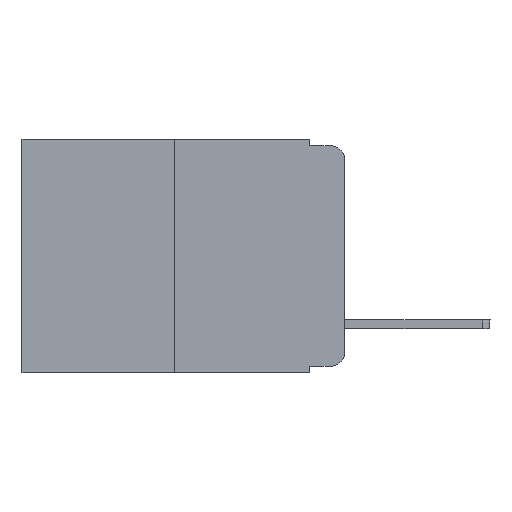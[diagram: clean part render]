
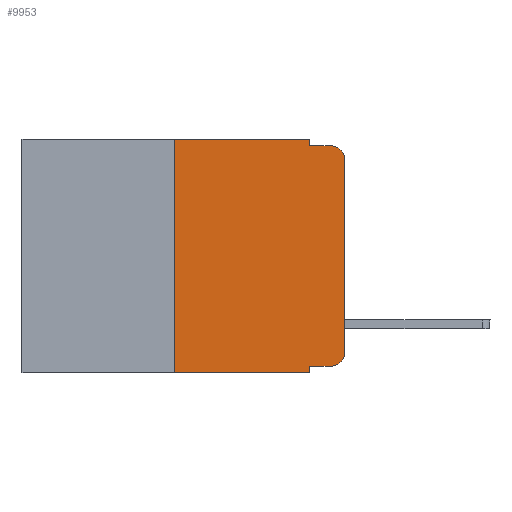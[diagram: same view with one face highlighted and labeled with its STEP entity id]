
A CAD part, left-side view. The second image highlights one B-rep face of the part: STEP entity #9953.
In plain terms, the highlighted planar face has unit normal (-1, 0, 0).
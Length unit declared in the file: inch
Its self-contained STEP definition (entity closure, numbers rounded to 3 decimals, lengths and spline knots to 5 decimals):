
#161 = CARTESIAN_POINT ( 'NONE',  ( 0., 0.473, 0. ) ) ;
#421 = DIRECTION ( 'NONE',  ( 0., -1., 0. ) ) ;
#553 = EDGE_CURVE ( 'NONE', #10030, #7135, #7659, .T. ) ;
#974 = VERTEX_POINT ( 'NONE', #9054 ) ;
#1174 = VERTEX_POINT ( 'NONE', #6200 ) ;
#1633 = ORIENTED_EDGE ( 'NONE', *, *, #19226, .T. ) ;
#1829 = DIRECTION ( 'NONE',  ( 0., 0., -1. ) ) ;
#1903 = VECTOR ( 'NONE', #6508, 39.37008 ) ;
#1920 = ORIENTED_EDGE ( 'NONE', *, *, #16495, .T. ) ;
#2309 = ORIENTED_EDGE ( 'NONE', *, *, #12067, .F. ) ;
#2712 = CARTESIAN_POINT ( 'NONE',  ( 0., 0.02, -0.03 ) ) ;
#3457 = EDGE_CURVE ( 'NONE', #1174, #17627, #9035, .T. ) ;
#3646 = CARTESIAN_POINT ( 'NONE',  ( 0., 0.051, -0.343 ) ) ;
#4109 = CARTESIAN_POINT ( 'NONE',  ( 0., 0.25, 0. ) ) ;
#4174 = CARTESIAN_POINT ( 'NONE',  ( 0., 0.051, -0.01 ) ) ;
#4301 = DIRECTION ( 'NONE',  ( 0., 0., -1. ) ) ;
#4708 = ORIENTED_EDGE ( 'NONE', *, *, #15659, .F. ) ;
#4810 = VERTEX_POINT ( 'NONE', #3646 ) ;
#5173 = VERTEX_POINT ( 'NONE', #8088 ) ;
#5210 = DIRECTION ( 'NONE',  ( 0., -1., 0. ) ) ;
#5859 = DIRECTION ( 'NONE',  ( 0., 0., -1. ) ) ;
#6125 = DIRECTION ( 'NONE',  ( -1., 0., 0. ) ) ;
#6200 = CARTESIAN_POINT ( 'NONE',  ( 0., 0.02, -0.333 ) ) ;
#6402 = CARTESIAN_POINT ( 'NONE',  ( 0., 0.051, -0.01 ) ) ;
#6508 = DIRECTION ( 'NONE',  ( 0., 0., 1. ) ) ;
#6717 = AXIS2_PLACEMENT_3D ( 'NONE', #2712, #20169, #4301 ) ;
#6783 = LINE ( 'NONE', #16011, #15188 ) ;
#6821 = ORIENTED_EDGE ( 'NONE', *, *, #12690, .T. ) ;
#7104 = CARTESIAN_POINT ( 'NONE',  ( 0., 0.051, 0. ) ) ;
#7135 = VERTEX_POINT ( 'NONE', #7104 ) ;
#7659 = LINE ( 'NONE', #161, #14336 ) ;
#7714 = CARTESIAN_POINT ( 'NONE',  ( 0., 0.051, -0.333 ) ) ;
#8065 = CARTESIAN_POINT ( 'NONE',  ( 0., 0.051, 0. ) ) ;
#8088 = CARTESIAN_POINT ( 'NONE',  ( 0., 0., -0.03 ) ) ;
#8226 = LINE ( 'NONE', #8065, #13408 ) ;
#8237 = CARTESIAN_POINT ( 'NONE',  ( 0., 0.051, -0.333 ) ) ;
#8518 = DIRECTION ( 'NONE',  ( 0., 0., -1. ) ) ;
#9035 = CIRCLE ( 'NONE', #12093, 0.02 ) ;
#9054 = CARTESIAN_POINT ( 'NONE',  ( 0., 0.25, -0.343 ) ) ;
#9237 = DIRECTION ( 'NONE',  ( 0., 0., -1. ) ) ;
#9323 = VERTEX_POINT ( 'NONE', #14420 ) ;
#9356 = ORIENTED_EDGE ( 'NONE', *, *, #20445, .F. ) ;
#9860 = DIRECTION ( 'NONE',  ( 0., -1., 0. ) ) ;
#9887 = EDGE_LOOP ( 'NONE', ( #6821, #1633, #10306, #4708, #19396, #9356, #1920, #2309, #15477, #16692 ) ) ;
#9953 = ADVANCED_FACE ( 'NONE', ( #17756 ), #10773, .F. ) ;
#10030 = VERTEX_POINT ( 'NONE', #4109 ) ;
#10306 = ORIENTED_EDGE ( 'NONE', *, *, #18862, .F. ) ;
#10563 = EDGE_CURVE ( 'NONE', #20033, #1174, #18745, .T. ) ;
#10773 = PLANE ( 'NONE',  #20268 ) ;
#11060 = VERTEX_POINT ( 'NONE', #4174 ) ;
#11178 = DIRECTION ( 'NONE',  ( 0., -1., 0. ) ) ;
#11866 = CIRCLE ( 'NONE', #6717, 0.02 ) ;
#11889 = VECTOR ( 'NONE', #11178, 39.37008 ) ;
#12067 = EDGE_CURVE ( 'NONE', #20033, #4810, #8226, .T. ) ;
#12093 = AXIS2_PLACEMENT_3D ( 'NONE', #20118, #6125, #9237 ) ;
#12411 = DIRECTION ( 'NONE',  ( 1., 0., 0. ) ) ;
#12690 = EDGE_CURVE ( 'NONE', #17627, #5173, #14129, .T. ) ;
#13100 = LINE ( 'NONE', #6402, #11889 ) ;
#13408 = VECTOR ( 'NONE', #1829, 39.37008 ) ;
#14129 = LINE ( 'NONE', #19614, #19874 ) ;
#14275 = LINE ( 'NONE', #14803, #20501 ) ;
#14336 = VECTOR ( 'NONE', #9860, 39.37008 ) ;
#14420 = CARTESIAN_POINT ( 'NONE',  ( 0., 0.02, -0.01 ) ) ;
#14491 = VECTOR ( 'NONE', #5210, 39.37008 ) ;
#14803 = CARTESIAN_POINT ( 'NONE',  ( 0., 0.051, 0. ) ) ;
#15188 = VECTOR ( 'NONE', #421, 39.37008 ) ;
#15477 = ORIENTED_EDGE ( 'NONE', *, *, #10563, .T. ) ;
#15659 = EDGE_CURVE ( 'NONE', #7135, #11060, #14275, .T. ) ;
#15993 = CARTESIAN_POINT ( 'NONE',  ( 0., 0.25, 0. ) ) ;
#16011 = CARTESIAN_POINT ( 'NONE',  ( 0., 0.473, -0.343 ) ) ;
#16261 = LINE ( 'NONE', #15993, #1903 ) ;
#16495 = EDGE_CURVE ( 'NONE', #974, #4810, #6783, .T. ) ;
#16692 = ORIENTED_EDGE ( 'NONE', *, *, #3457, .T. ) ;
#17061 = CARTESIAN_POINT ( 'NONE',  ( 0., 0.473, 0. ) ) ;
#17627 = VERTEX_POINT ( 'NONE', #19188 ) ;
#17756 = FACE_OUTER_BOUND ( 'NONE', #9887, .T. ) ;
#18745 = LINE ( 'NONE', #8237, #14491 ) ;
#18862 = EDGE_CURVE ( 'NONE', #11060, #9323, #13100, .T. ) ;
#19188 = CARTESIAN_POINT ( 'NONE',  ( 0., 0., -0.313 ) ) ;
#19226 = EDGE_CURVE ( 'NONE', #5173, #9323, #11866, .T. ) ;
#19396 = ORIENTED_EDGE ( 'NONE', *, *, #553, .F. ) ;
#19417 = DIRECTION ( 'NONE',  ( 0., 0., 1. ) ) ;
#19614 = CARTESIAN_POINT ( 'NONE',  ( 0., 0., 0. ) ) ;
#19874 = VECTOR ( 'NONE', #19417, 39.37008 ) ;
#20033 = VERTEX_POINT ( 'NONE', #7714 ) ;
#20118 = CARTESIAN_POINT ( 'NONE',  ( 0., 0.02, -0.313 ) ) ;
#20169 = DIRECTION ( 'NONE',  ( -1., 0., 0. ) ) ;
#20268 = AXIS2_PLACEMENT_3D ( 'NONE', #17061, #12411, #5859 ) ;
#20445 = EDGE_CURVE ( 'NONE', #974, #10030, #16261, .T. ) ;
#20501 = VECTOR ( 'NONE', #8518, 39.37008 ) ;
